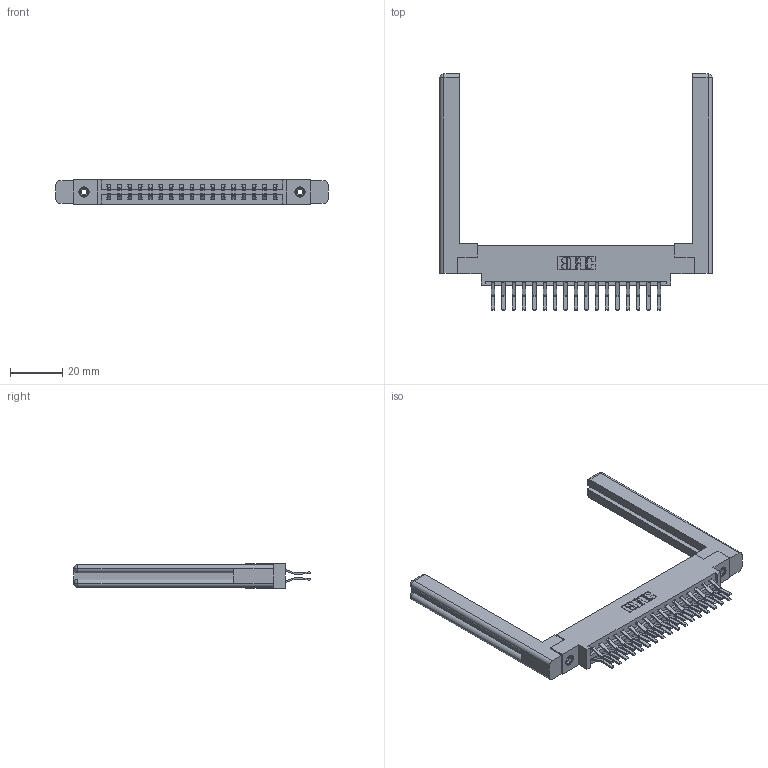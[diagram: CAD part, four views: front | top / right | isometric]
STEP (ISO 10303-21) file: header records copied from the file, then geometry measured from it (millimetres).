
FILE_DESCRIPTION (( 'STEP AP203' ), '1' );
FILE_NAME ('387-034-560-858.STEP', '2019-10-17T18:34:44', ( '' ), ( '' ), 'SwSTEP 2.0', 'SolidWorks 2016', '' );
FILE_SCHEMA (( 'CONFIG_CONTROL_DESIGN' ));
Length unit declared in the file: inch
Products named in the file (5): 307-220-058; 337 Part_0.170 Offset - 0.156 Dia-TI; 387-034-560-858; 345-250-001_345-250-001-102; 345-292-001_560 Tail
Assembly tree (39 placements, depth 2):
  387-034-560-858
    337 Part_0.170 Offset - 0.156 Dia-TI
    345-292-001_560 Tail  x34
    345-250-001_345-250-001-102  x2
    307-220-058  x2
Bounding box: 103.99 x 90.19 x 9.4 mm (x, y, z)
Volume: 17874 mm3; surface area: 17688.9 mm2
Topology: 39 solids, 39 shells, 2164 faces, 6355 edges, 4178 vertices
Faces by surface type: plane 1450, cylinder 690, cone 12, torus 12
Entity records: 19268 total; most frequent: CARTESIAN_POINT 3277, ORIENTED_EDGE 3152, DIRECTION 2852, EDGE_CURVE 1576, VECTOR 1396, LINE 1396, VERTEX_POINT 1042, AXIS2_PLACEMENT_3D 728
